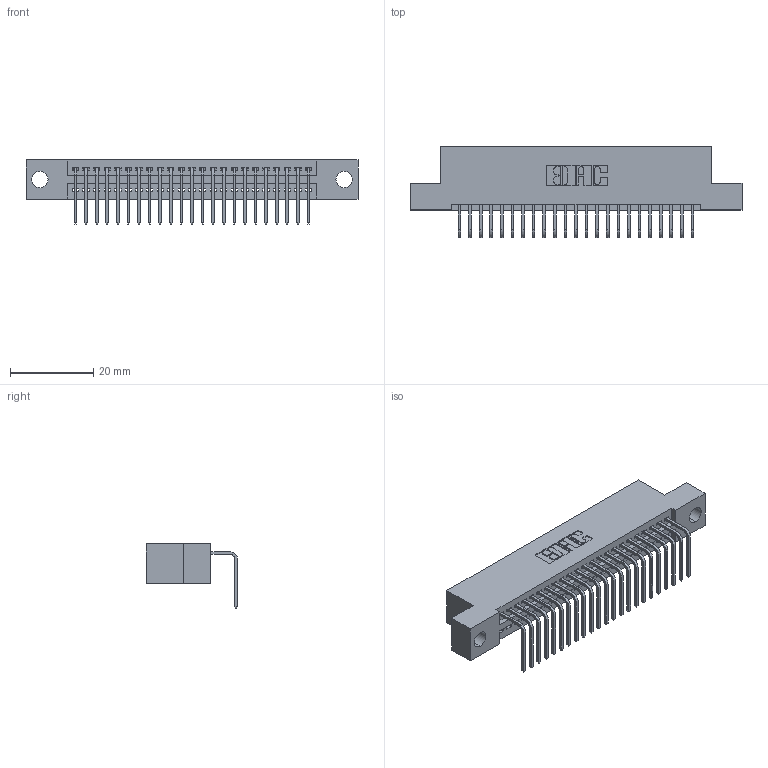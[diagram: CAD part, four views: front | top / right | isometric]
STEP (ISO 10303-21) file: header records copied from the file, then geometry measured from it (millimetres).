
FILE_DESCRIPTION (( 'STEP AP203' ), '1' );
FILE_NAME ('345-023-558-104.STEP', '2021-06-09T16:13:46', ( '' ), ( '' ), 'SwSTEP 2.0', 'SolidWorks 2020', '' );
FILE_SCHEMA (( 'CONFIG_CONTROL_DESIGN' ));
Length unit declared in the file: inch
Products named in the file (3): 345 Part_Flush Mounting Lugs - 0.156 Dia-TI; 345-023-558-104; 345-292-001_558 Tail - 2
Assembly tree (24 placements, depth 2):
  345-023-558-104
    345 Part_Flush Mounting Lugs - 0.156 Dia-TI
    345-292-001_558 Tail - 2  x23
Bounding box: 79.63 x 21.83 x 15.37 mm (x, y, z)
Volume: 7378.3 mm3; surface area: 9839.6 mm2
Topology: 24 solids, 24 shells, 1520 faces, 4563 edges, 3010 vertices
Faces by surface type: plane 1060, cylinder 460
Entity records: 20371 total; most frequent: CARTESIAN_POINT 3539, ORIENTED_EDGE 3494, DIRECTION 3117, EDGE_CURVE 1747, LINE 1523, VECTOR 1523, VERTEX_POINT 1162, AXIS2_PLACEMENT_3D 797
